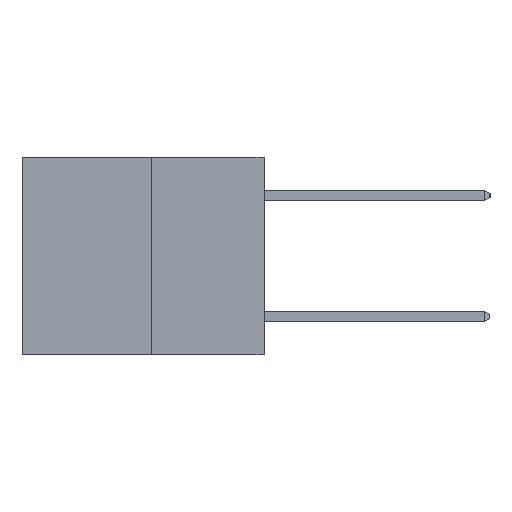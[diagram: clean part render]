
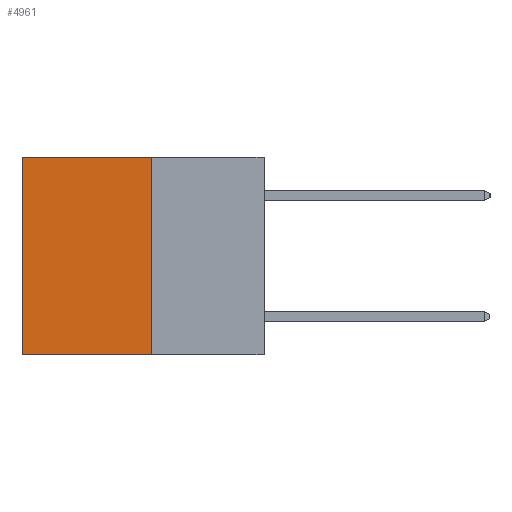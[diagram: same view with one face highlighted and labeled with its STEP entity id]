
A CAD part, left-side view. The second image highlights one B-rep face of the part: STEP entity #4961.
In plain terms, the highlighted planar face has unit normal (-1, 0, 0).
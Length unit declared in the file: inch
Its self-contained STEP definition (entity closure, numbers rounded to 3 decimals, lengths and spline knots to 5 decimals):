
#739 = EDGE_CURVE ( 'NONE', #4018, #6669, #7063, .T. ) ;
#745 = CARTESIAN_POINT ( 'NONE',  ( 0.3165, 0.28, -0.49 ) ) ;
#1074 = CARTESIAN_POINT ( 'NONE',  ( 0.3165, 0.28, -0.49 ) ) ;
#1133 = VECTOR ( 'NONE', #3916, 39.37008 ) ;
#1416 = FACE_OUTER_BOUND ( 'NONE', #4176, .T. ) ;
#1906 = ORIENTED_EDGE ( 'NONE', *, *, #7291, .T. ) ;
#2037 = VECTOR ( 'NONE', #10993, 39.37008 ) ;
#2216 = CARTESIAN_POINT ( 'NONE',  ( 0.3165, 0.28, -0.49 ) ) ;
#2360 = ORIENTED_EDGE ( 'NONE', *, *, #10846, .F. ) ;
#2662 = CARTESIAN_POINT ( 'NONE',  ( 0.3165, 0.28, 0. ) ) ;
#2916 = CARTESIAN_POINT ( 'NONE',  ( 0.3165, 0.28, 0. ) ) ;
#3040 = LINE ( 'NONE', #2916, #10290 ) ;
#3190 = EDGE_CURVE ( 'NONE', #3666, #10739, #3040, .T. ) ;
#3548 = PLANE ( 'NONE',  #5483 ) ;
#3666 = VERTEX_POINT ( 'NONE', #2662 ) ;
#3710 = CARTESIAN_POINT ( 'NONE',  ( 0.3165, 0.6, 0. ) ) ;
#3916 = DIRECTION ( 'NONE',  ( 0., 0., -1. ) ) ;
#4006 = ORIENTED_EDGE ( 'NONE', *, *, #3190, .T. ) ;
#4018 = VERTEX_POINT ( 'NONE', #2216 ) ;
#4176 = EDGE_LOOP ( 'NONE', ( #1906, #7077, #2360, #4006 ) ) ;
#4450 = CARTESIAN_POINT ( 'NONE',  ( 0.3165, 0.28, -0.49 ) ) ;
#4961 = ADVANCED_FACE ( 'NONE', ( #1416 ), #3548, .F. ) ;
#5076 = LINE ( 'NONE', #9449, #1133 ) ;
#5483 = AXIS2_PLACEMENT_3D ( 'NONE', #4450, #6368, #10843 ) ;
#5505 = CARTESIAN_POINT ( 'NONE',  ( 0.3165, 0.6, -0.49 ) ) ;
#6255 = VECTOR ( 'NONE', #10488, 39.37008 ) ;
#6368 = DIRECTION ( 'NONE',  ( 1., 0., 0. ) ) ;
#6669 = VERTEX_POINT ( 'NONE', #5505 ) ;
#7063 = LINE ( 'NONE', #745, #2037 ) ;
#7077 = ORIENTED_EDGE ( 'NONE', *, *, #739, .F. ) ;
#7291 = EDGE_CURVE ( 'NONE', #10739, #6669, #5076, .T. ) ;
#8745 = LINE ( 'NONE', #1074, #6255 ) ;
#9449 = CARTESIAN_POINT ( 'NONE',  ( 0.3165, 0.6, -0.49 ) ) ;
#10290 = VECTOR ( 'NONE', #11439, 39.37008 ) ;
#10488 = DIRECTION ( 'NONE',  ( 0., 0., -1. ) ) ;
#10739 = VERTEX_POINT ( 'NONE', #3710 ) ;
#10843 = DIRECTION ( 'NONE',  ( 0., 0., -1. ) ) ;
#10846 = EDGE_CURVE ( 'NONE', #3666, #4018, #8745, .T. ) ;
#10993 = DIRECTION ( 'NONE',  ( 0., 1., 0. ) ) ;
#11439 = DIRECTION ( 'NONE',  ( 0., 1., 0. ) ) ;
